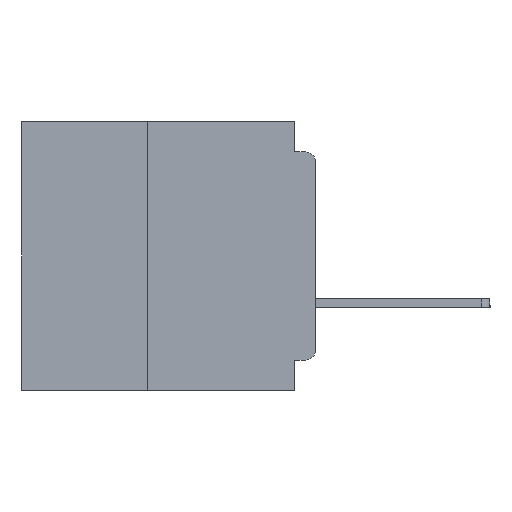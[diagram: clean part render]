
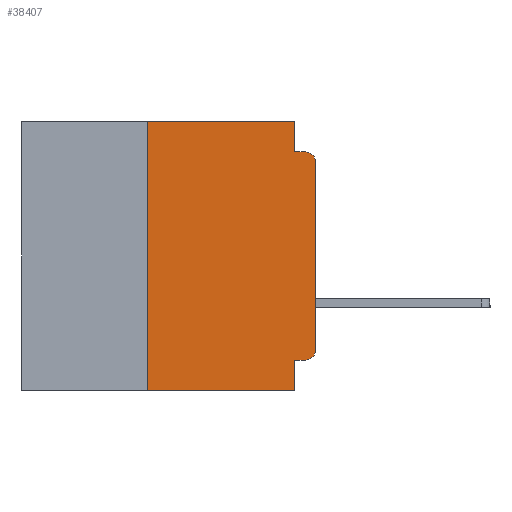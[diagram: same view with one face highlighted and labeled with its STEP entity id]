
A CAD part, left-side view. The second image highlights one B-rep face of the part: STEP entity #38407.
In plain terms, the highlighted planar face has unit normal (-1, 0, 0).
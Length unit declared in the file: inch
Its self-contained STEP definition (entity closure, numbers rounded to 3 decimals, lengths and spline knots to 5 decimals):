
#421 = CIRCLE ( 'NONE', #19208, 0.015 ) ;
#1318 = CARTESIAN_POINT ( 'NONE',  ( 0., 0.015, -0.045 ) ) ;
#1369 = VECTOR ( 'NONE', #19161, 39.37008 ) ;
#2133 = VERTEX_POINT ( 'NONE', #25442 ) ;
#2795 = DIRECTION ( 'NONE',  ( 0., 0., -1. ) ) ;
#3563 = DIRECTION ( 'NONE',  ( 0., 1., 0. ) ) ;
#3888 = VECTOR ( 'NONE', #33654, 39.37008 ) ;
#4361 = CARTESIAN_POINT ( 'NONE',  ( 0., 0., -0.06 ) ) ;
#4383 = CARTESIAN_POINT ( 'NONE',  ( 0., 0., 0. ) ) ;
#4668 = LINE ( 'NONE', #18653, #21599 ) ;
#4873 = LINE ( 'NONE', #30448, #3888 ) ;
#4995 = EDGE_CURVE ( 'NONE', #34335, #10761, #6835, .T. ) ;
#5199 = LINE ( 'NONE', #30012, #20125 ) ;
#6294 = VERTEX_POINT ( 'NONE', #18301 ) ;
#6629 = LINE ( 'NONE', #36756, #22522 ) ;
#6835 = CIRCLE ( 'NONE', #22233, 0.015 ) ;
#7529 = DIRECTION ( 'NONE',  ( 1., 0., 0. ) ) ;
#7593 = DIRECTION ( 'NONE',  ( 0., 0., 1. ) ) ;
#8315 = CARTESIAN_POINT ( 'NONE',  ( 0., 0.25, -0.4 ) ) ;
#8415 = VERTEX_POINT ( 'NONE', #4361 ) ;
#8916 = CARTESIAN_POINT ( 'NONE',  ( 0., 0., -0.34 ) ) ;
#9860 = LINE ( 'NONE', #15972, #1369 ) ;
#10593 = PLANE ( 'NONE',  #35746 ) ;
#10645 = VERTEX_POINT ( 'NONE', #11575 ) ;
#10749 = EDGE_CURVE ( 'NONE', #8415, #12996, #421, .T. ) ;
#10761 = VERTEX_POINT ( 'NONE', #8916 ) ;
#10771 = EDGE_LOOP ( 'NONE', ( #39120, #17402, #33625, #19067, #25006, #17053, #15449, #27867, #25512, #32476 ) ) ;
#11523 = CARTESIAN_POINT ( 'NONE',  ( 0., 0.015, -0.355 ) ) ;
#11575 = CARTESIAN_POINT ( 'NONE',  ( 0., 0.031, -0.045 ) ) ;
#12977 = EDGE_CURVE ( 'NONE', #10761, #8415, #14181, .T. ) ;
#12996 = VERTEX_POINT ( 'NONE', #1318 ) ;
#13046 = CARTESIAN_POINT ( 'NONE',  ( 0., 0., -0.355 ) ) ;
#14181 = LINE ( 'NONE', #4383, #29027 ) ;
#15323 = CARTESIAN_POINT ( 'NONE',  ( 0., 0.015, -0.06 ) ) ;
#15366 = EDGE_CURVE ( 'NONE', #34335, #2133, #40032, .T. ) ;
#15449 = ORIENTED_EDGE ( 'NONE', *, *, #16443, .T. ) ;
#15972 = CARTESIAN_POINT ( 'NONE',  ( 0., 0., -0.045 ) ) ;
#16234 = EDGE_CURVE ( 'NONE', #23338, #6294, #5199, .T. ) ;
#16443 = EDGE_CURVE ( 'NONE', #23338, #39246, #4668, .T. ) ;
#17053 = ORIENTED_EDGE ( 'NONE', *, *, #16234, .F. ) ;
#17402 = ORIENTED_EDGE ( 'NONE', *, *, #10749, .T. ) ;
#17536 = DIRECTION ( 'NONE',  ( 0., 0., 1. ) ) ;
#18301 = CARTESIAN_POINT ( 'NONE',  ( 0., 0.25, 0. ) ) ;
#18519 = DIRECTION ( 'NONE',  ( 0., 0., -1. ) ) ;
#18653 = CARTESIAN_POINT ( 'NONE',  ( 0., 0.437, -0.4 ) ) ;
#19067 = ORIENTED_EDGE ( 'NONE', *, *, #23306, .F. ) ;
#19161 = DIRECTION ( 'NONE',  ( 0., -1., 0. ) ) ;
#19208 = AXIS2_PLACEMENT_3D ( 'NONE', #15323, #37505, #18519 ) ;
#20125 = VECTOR ( 'NONE', #17536, 39.37008 ) ;
#20595 = EDGE_CURVE ( 'NONE', #10645, #12996, #9860, .T. ) ;
#21599 = VECTOR ( 'NONE', #40768, 39.37008 ) ;
#21674 = DIRECTION ( 'NONE',  ( 0., 0., -1. ) ) ;
#21707 = DIRECTION ( 'NONE',  ( -1., 0., 0. ) ) ;
#21714 = CARTESIAN_POINT ( 'NONE',  ( 0., 0.015, -0.34 ) ) ;
#22233 = AXIS2_PLACEMENT_3D ( 'NONE', #21714, #21707, #21674 ) ;
#22522 = VECTOR ( 'NONE', #39938, 39.37008 ) ;
#23306 = EDGE_CURVE ( 'NONE', #38690, #10645, #6629, .T. ) ;
#23338 = VERTEX_POINT ( 'NONE', #8315 ) ;
#23683 = LINE ( 'NONE', #40782, #39571 ) ;
#25006 = ORIENTED_EDGE ( 'NONE', *, *, #39643, .F. ) ;
#25442 = CARTESIAN_POINT ( 'NONE',  ( 0., 0.031, -0.355 ) ) ;
#25512 = ORIENTED_EDGE ( 'NONE', *, *, #15366, .F. ) ;
#26529 = CARTESIAN_POINT ( 'NONE',  ( 0., 0.437, 0. ) ) ;
#27867 = ORIENTED_EDGE ( 'NONE', *, *, #40422, .F. ) ;
#29027 = VECTOR ( 'NONE', #7593, 39.37008 ) ;
#29715 = DIRECTION ( 'NONE',  ( 0., 0., -1. ) ) ;
#30012 = CARTESIAN_POINT ( 'NONE',  ( 0., 0.25, -0.4 ) ) ;
#30448 = CARTESIAN_POINT ( 'NONE',  ( 0., 0.437, 0. ) ) ;
#31594 = VECTOR ( 'NONE', #3563, 39.37008 ) ;
#32476 = ORIENTED_EDGE ( 'NONE', *, *, #4995, .T. ) ;
#33625 = ORIENTED_EDGE ( 'NONE', *, *, #20595, .F. ) ;
#33654 = DIRECTION ( 'NONE',  ( 0., -1., 0. ) ) ;
#34106 = CARTESIAN_POINT ( 'NONE',  ( 0., 0.031, -0.4 ) ) ;
#34335 = VERTEX_POINT ( 'NONE', #11523 ) ;
#35746 = AXIS2_PLACEMENT_3D ( 'NONE', #26529, #7529, #29715 ) ;
#36756 = CARTESIAN_POINT ( 'NONE',  ( 0., 0.031, 0. ) ) ;
#37505 = DIRECTION ( 'NONE',  ( -1., 0., 0. ) ) ;
#37842 = FACE_OUTER_BOUND ( 'NONE', #10771, .T. ) ;
#38407 = ADVANCED_FACE ( 'NONE', ( #37842 ), #10593, .F. ) ;
#38690 = VERTEX_POINT ( 'NONE', #40500 ) ;
#39120 = ORIENTED_EDGE ( 'NONE', *, *, #12977, .T. ) ;
#39246 = VERTEX_POINT ( 'NONE', #34106 ) ;
#39571 = VECTOR ( 'NONE', #2795, 39.37008 ) ;
#39643 = EDGE_CURVE ( 'NONE', #6294, #38690, #4873, .T. ) ;
#39938 = DIRECTION ( 'NONE',  ( 0., 0., -1. ) ) ;
#40032 = LINE ( 'NONE', #13046, #31594 ) ;
#40422 = EDGE_CURVE ( 'NONE', #2133, #39246, #23683, .T. ) ;
#40500 = CARTESIAN_POINT ( 'NONE',  ( 0., 0.031, 0. ) ) ;
#40768 = DIRECTION ( 'NONE',  ( 0., -1., 0. ) ) ;
#40782 = CARTESIAN_POINT ( 'NONE',  ( 0., 0.031, -0.4 ) ) ;
